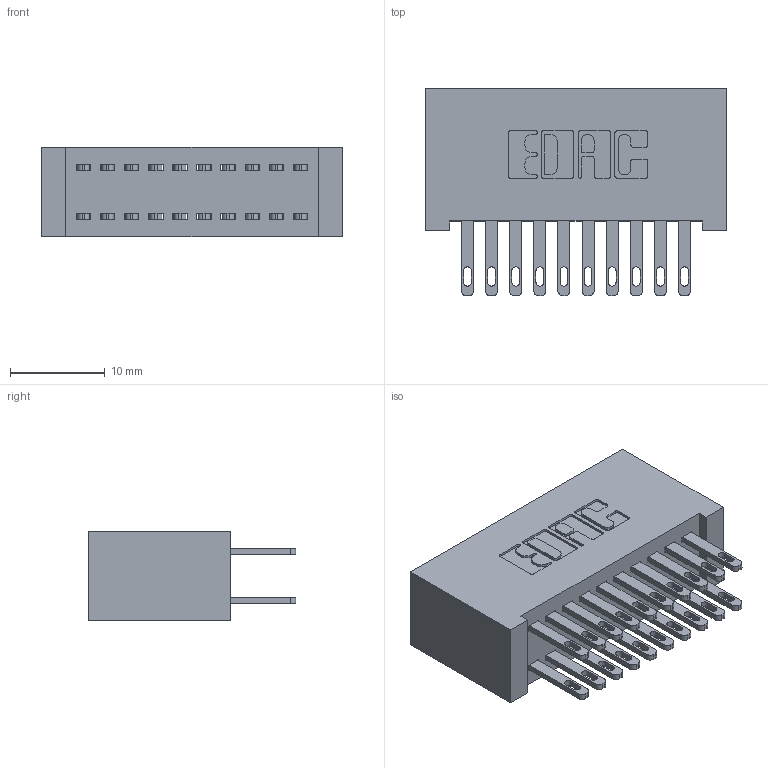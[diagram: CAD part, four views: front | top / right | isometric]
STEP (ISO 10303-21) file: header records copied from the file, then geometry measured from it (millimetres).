
FILE_DESCRIPTION (( 'STEP AP203' ), '1' );
FILE_NAME ('892-020-500-201.STEP', '2020-09-21T13:56:16', ( '' ), ( '' ), 'SwSTEP 2.0', 'SolidWorks 2020', '' );
FILE_SCHEMA (( 'CONFIG_CONTROL_DESIGN' ));
Length unit declared in the file: inch
Products named in the file (3): 842 Part_Lugless; 345-292-001_345-293-100; 892-020-500-201
Assembly tree (21 placements, depth 2):
  892-020-500-201
    842 Part_Lugless
    345-292-001_345-293-100  x20
Bounding box: 31.65 x 21.85 x 9.4 mm (x, y, z)
Volume: 3192.8 mm3; surface area: 5046.2 mm2
Topology: 21 solids, 21 shells, 1062 faces, 3215 edges, 2142 vertices
Faces by surface type: plane 662, cylinder 400
Entity records: 10093 total; most frequent: CARTESIAN_POINT 1706, ORIENTED_EDGE 1642, DIRECTION 1509, EDGE_CURVE 821, VECTOR 697, LINE 697, VERTEX_POINT 546, AXIS2_PLACEMENT_3D 406
